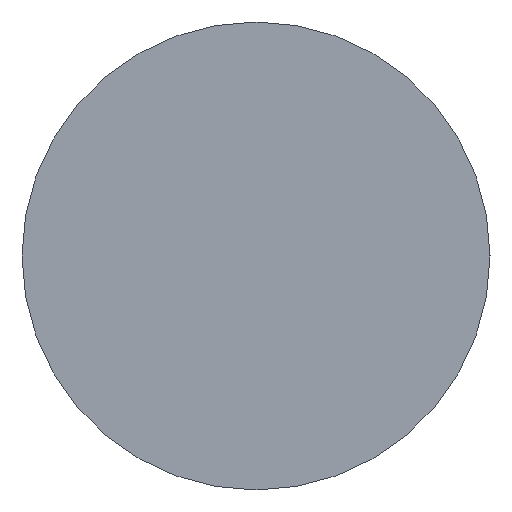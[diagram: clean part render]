
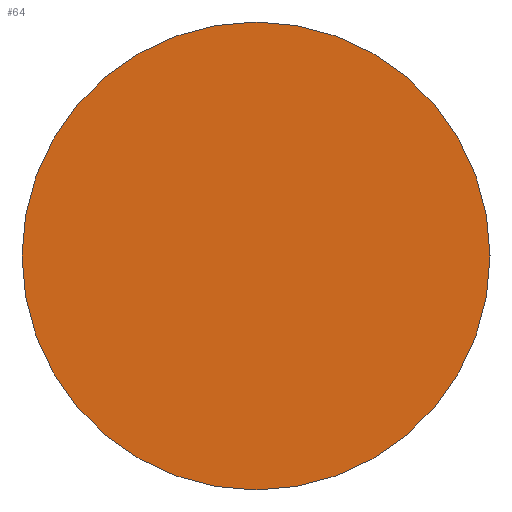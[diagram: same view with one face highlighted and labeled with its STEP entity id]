
A CAD part, left-side view. The second image highlights one B-rep face of the part: STEP entity #64.
In plain terms, the highlighted planar face has unit normal (-1, 0, 0).
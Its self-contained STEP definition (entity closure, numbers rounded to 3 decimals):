
#17 = DIRECTION ( 'NONE',  ( 0., 0., -1. ) ) ;
#19 = DIRECTION ( 'NONE',  ( 1., 0., 0. ) ) ;
#24 = CARTESIAN_POINT ( 'NONE',  ( -5., 0., 0. ) ) ;
#30 = CARTESIAN_POINT ( 'NONE',  ( -5., 0., 0. ) ) ;
#44 = AXIS2_PLACEMENT_3D ( 'NONE', #24, #19, #17 ) ;
#51 = AXIS2_PLACEMENT_3D ( 'NONE', #30, #69, #65 ) ;
#52 = AXIS2_PLACEMENT_3D ( 'NONE', #126, #123, #122 ) ;
#56 = VERTEX_POINT ( 'NONE', #79 ) ;
#60 = ORIENTED_EDGE ( 'NONE', *, *, #132, .F. ) ;
#61 = EDGE_LOOP ( 'NONE', ( #60, #119 ) ) ;
#64 = ADVANCED_FACE ( 'NONE', ( #81 ), #125, .F. ) ;
#65 = DIRECTION ( 'NONE',  ( 0., 0., -1. ) ) ;
#69 = DIRECTION ( 'NONE',  ( 1., 0., 0. ) ) ;
#72 = CIRCLE ( 'NONE', #44, 3.125 ) ;
#76 = CIRCLE ( 'NONE', #51, 3.125 ) ;
#79 = CARTESIAN_POINT ( 'NONE',  ( -5., 0., -3.125 ) ) ;
#81 = FACE_OUTER_BOUND ( 'NONE', #61, .T. ) ;
#89 = VERTEX_POINT ( 'NONE', #92 ) ;
#92 = CARTESIAN_POINT ( 'NONE',  ( -5., 0., 3.125 ) ) ;
#104 = EDGE_CURVE ( 'NONE', #56, #89, #76, .T. ) ;
#119 = ORIENTED_EDGE ( 'NONE', *, *, #104, .F. ) ;
#122 = DIRECTION ( 'NONE',  ( 0., 0., -1. ) ) ;
#123 = DIRECTION ( 'NONE',  ( 1., 0., 0. ) ) ;
#125 = PLANE ( 'NONE',  #52 ) ;
#126 = CARTESIAN_POINT ( 'NONE',  ( -5., 0., 0. ) ) ;
#132 = EDGE_CURVE ( 'NONE', #89, #56, #72, .T. ) ;
